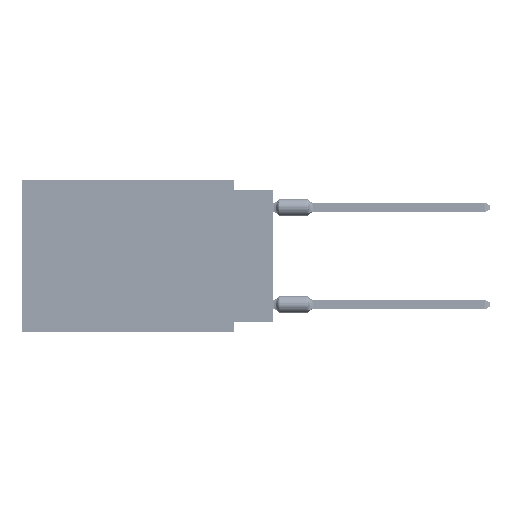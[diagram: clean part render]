
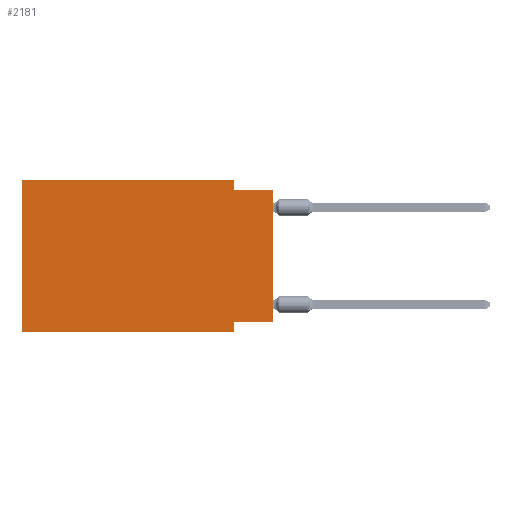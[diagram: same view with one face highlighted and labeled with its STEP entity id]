
A CAD part, left-side view. The second image highlights one B-rep face of the part: STEP entity #2181.
In plain terms, the highlighted planar face has unit normal (-1, 0, 0).
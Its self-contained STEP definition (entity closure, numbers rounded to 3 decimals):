
#488 = DIRECTION ( 'NONE',  ( 0., 0., -1. ) ) ;
#2093 = AXIS2_PLACEMENT_3D ( 'NONE', #42281, #67450, #15475 ) ;
#2181 = ADVANCED_FACE ( 'NONE', ( #21669 ), #79865, .F. ) ;
#5321 = VERTEX_POINT ( 'NONE', #47544 ) ;
#5766 = VERTEX_POINT ( 'NONE', #72243 ) ;
#6561 = VERTEX_POINT ( 'NONE', #65036 ) ;
#6953 = VECTOR ( 'NONE', #59853, 1000. ) ;
#8677 = VECTOR ( 'NONE', #79075, 1000. ) ;
#9051 = CARTESIAN_POINT ( 'NONE',  ( 0., 16.383, 0. ) ) ;
#9738 = ORIENTED_EDGE ( 'NONE', *, *, #11901, .F. ) ;
#10513 = ORIENTED_EDGE ( 'NONE', *, *, #58466, .T. ) ;
#11493 = LINE ( 'NONE', #36678, #28005 ) ;
#11901 = EDGE_CURVE ( 'NONE', #68314, #75146, #28865, .T. ) ;
#12031 = CARTESIAN_POINT ( 'NONE',  ( 0., 16.383, 0. ) ) ;
#12271 = VECTOR ( 'NONE', #488, 1000. ) ;
#13486 = ORIENTED_EDGE ( 'NONE', *, *, #66671, .F. ) ;
#13933 = VECTOR ( 'NONE', #58918, 1000. ) ;
#15097 = EDGE_CURVE ( 'NONE', #5766, #53597, #30188, .T. ) ;
#15475 = DIRECTION ( 'NONE',  ( 0., 0., -1. ) ) ;
#17321 = ORIENTED_EDGE ( 'NONE', *, *, #28173, .F. ) ;
#17451 = ORIENTED_EDGE ( 'NONE', *, *, #63010, .F. ) ;
#21669 = FACE_OUTER_BOUND ( 'NONE', #61217, .T. ) ;
#23319 = LINE ( 'NONE', #66658, #8677 ) ;
#25135 = CARTESIAN_POINT ( 'NONE',  ( 0., 2.54, 0. ) ) ;
#25142 = VERTEX_POINT ( 'NONE', #25135 ) ;
#25689 = VERTEX_POINT ( 'NONE', #45640 ) ;
#26716 = LINE ( 'NONE', #45702, #13933 ) ;
#27108 = LINE ( 'NONE', #52279, #65258 ) ;
#28005 = VECTOR ( 'NONE', #61858, 1000. ) ;
#28173 = EDGE_CURVE ( 'NONE', #53597, #25142, #23319, .T. ) ;
#28865 = LINE ( 'NONE', #65627, #6953 ) ;
#30188 = LINE ( 'NONE', #12031, #32354 ) ;
#30226 = LINE ( 'NONE', #68215, #12271 ) ;
#32354 = VECTOR ( 'NONE', #62406, 1000. ) ;
#36095 = LINE ( 'NONE', #48880, #53973 ) ;
#36499 = DIRECTION ( 'NONE',  ( 0., -1., 0. ) ) ;
#36678 = CARTESIAN_POINT ( 'NONE',  ( 0., 0., -0.635 ) ) ;
#42281 = CARTESIAN_POINT ( 'NONE',  ( 0., 16.383, 0. ) ) ;
#43726 = ORIENTED_EDGE ( 'NONE', *, *, #47316, .F. ) ;
#45640 = CARTESIAN_POINT ( 'NONE',  ( 0., 2.54, -9.906 ) ) ;
#45702 = CARTESIAN_POINT ( 'NONE',  ( 0., 2.54, 0. ) ) ;
#47316 = EDGE_CURVE ( 'NONE', #5321, #6561, #11493, .T. ) ;
#47544 = CARTESIAN_POINT ( 'NONE',  ( 0., 2.54, -0.635 ) ) ;
#48880 = CARTESIAN_POINT ( 'NONE',  ( 0., 16.383, -9.906 ) ) ;
#51952 = CARTESIAN_POINT ( 'NONE',  ( 0., 0., -9.271 ) ) ;
#52279 = CARTESIAN_POINT ( 'NONE',  ( 0., 0., 0. ) ) ;
#52578 = CARTESIAN_POINT ( 'NONE',  ( 0., 2.54, -9.271 ) ) ;
#53597 = VERTEX_POINT ( 'NONE', #9051 ) ;
#53973 = VECTOR ( 'NONE', #36499, 1000. ) ;
#58466 = EDGE_CURVE ( 'NONE', #5766, #25689, #36095, .T. ) ;
#58918 = DIRECTION ( 'NONE',  ( 0., 0., -1. ) ) ;
#59853 = DIRECTION ( 'NONE',  ( 0., 1., 0. ) ) ;
#61217 = EDGE_LOOP ( 'NONE', ( #75253, #43726, #13486, #17321, #69923, #10513, #17451, #9738 ) ) ;
#61858 = DIRECTION ( 'NONE',  ( 0., -1., 0. ) ) ;
#62406 = DIRECTION ( 'NONE',  ( 0., 0., 1. ) ) ;
#63010 = EDGE_CURVE ( 'NONE', #75146, #25689, #30226, .T. ) ;
#65036 = CARTESIAN_POINT ( 'NONE',  ( 0., 0., -0.635 ) ) ;
#65258 = VECTOR ( 'NONE', #77490, 1000. ) ;
#65409 = EDGE_CURVE ( 'NONE', #68314, #6561, #27108, .T. ) ;
#65627 = CARTESIAN_POINT ( 'NONE',  ( 0., 0., -9.271 ) ) ;
#66658 = CARTESIAN_POINT ( 'NONE',  ( 0., 16.383, 0. ) ) ;
#66671 = EDGE_CURVE ( 'NONE', #25142, #5321, #26716, .T. ) ;
#67450 = DIRECTION ( 'NONE',  ( 1., 0., 0. ) ) ;
#68215 = CARTESIAN_POINT ( 'NONE',  ( 0., 2.54, -9.906 ) ) ;
#68314 = VERTEX_POINT ( 'NONE', #51952 ) ;
#69923 = ORIENTED_EDGE ( 'NONE', *, *, #15097, .F. ) ;
#72243 = CARTESIAN_POINT ( 'NONE',  ( 0., 16.383, -9.906 ) ) ;
#75146 = VERTEX_POINT ( 'NONE', #52578 ) ;
#75253 = ORIENTED_EDGE ( 'NONE', *, *, #65409, .T. ) ;
#77490 = DIRECTION ( 'NONE',  ( 0., 0., 1. ) ) ;
#79075 = DIRECTION ( 'NONE',  ( 0., -1., 0. ) ) ;
#79865 = PLANE ( 'NONE',  #2093 ) ;
